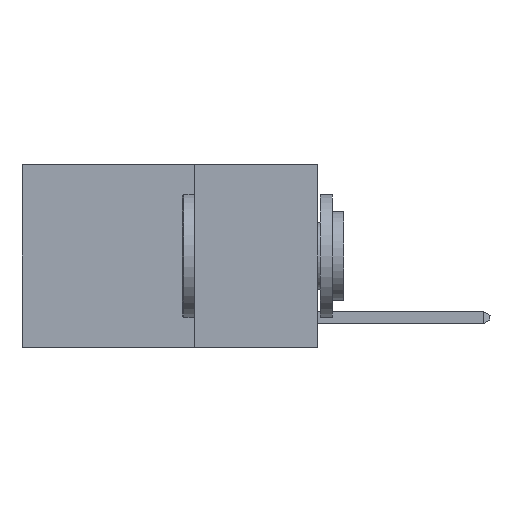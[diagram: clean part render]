
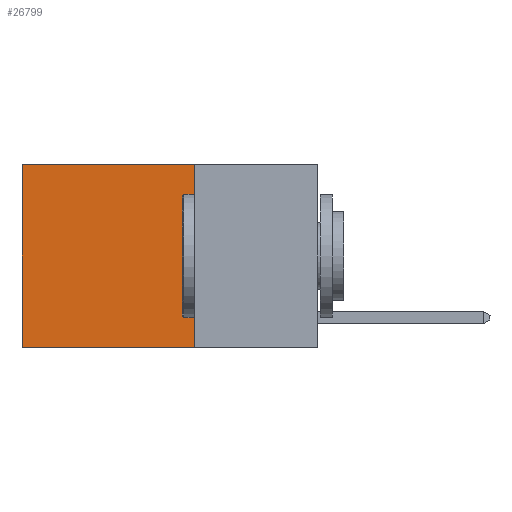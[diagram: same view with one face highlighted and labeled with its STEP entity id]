
A CAD part, left-side view. The second image highlights one B-rep face of the part: STEP entity #26799.
In plain terms, the highlighted planar face has unit normal (-1, 0, 0).
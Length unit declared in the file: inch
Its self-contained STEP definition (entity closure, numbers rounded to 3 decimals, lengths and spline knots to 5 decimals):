
#865 = VERTEX_POINT ( 'NONE', #9514 ) ;
#1272 = CARTESIAN_POINT ( 'NONE',  ( 0.2625, 0.25, -0.37 ) ) ;
#1354 = VECTOR ( 'NONE', #16297, 39.37008 ) ;
#2246 = LINE ( 'NONE', #26280, #8430 ) ;
#4531 = DIRECTION ( 'NONE',  ( 0., 1., 0. ) ) ;
#5643 = VERTEX_POINT ( 'NONE', #23526 ) ;
#7073 = ORIENTED_EDGE ( 'NONE', *, *, #19416, .T. ) ;
#7747 = LINE ( 'NONE', #10006, #25312 ) ;
#8430 = VECTOR ( 'NONE', #4531, 39.37008 ) ;
#8910 = EDGE_CURVE ( 'NONE', #5643, #9985, #27358, .T. ) ;
#9514 = CARTESIAN_POINT ( 'NONE',  ( 0.2625, 0.6, 0. ) ) ;
#9985 = VERTEX_POINT ( 'NONE', #1272 ) ;
#10006 = CARTESIAN_POINT ( 'NONE',  ( 0.2625, 0.25, 0. ) ) ;
#11448 = DIRECTION ( 'NONE',  ( 0., 0., -1. ) ) ;
#13441 = PLANE ( 'NONE',  #13718 ) ;
#13718 = AXIS2_PLACEMENT_3D ( 'NONE', #21730, #15724, #11448 ) ;
#15724 = DIRECTION ( 'NONE',  ( 1., 0., 0. ) ) ;
#16297 = DIRECTION ( 'NONE',  ( 0., 0., -1. ) ) ;
#16443 = DIRECTION ( 'NONE',  ( 0., 1., 0. ) ) ;
#16585 = ORIENTED_EDGE ( 'NONE', *, *, #24616, .T. ) ;
#19061 = CARTESIAN_POINT ( 'NONE',  ( 0.2625, 0.6, -0.37 ) ) ;
#19230 = CARTESIAN_POINT ( 'NONE',  ( 0.2625, 0.6, 0. ) ) ;
#19380 = DIRECTION ( 'NONE',  ( 0., 0., -1. ) ) ;
#19416 = EDGE_CURVE ( 'NONE', #865, #23533, #21373, .T. ) ;
#19991 = ORIENTED_EDGE ( 'NONE', *, *, #23078, .F. ) ;
#21373 = LINE ( 'NONE', #19230, #24421 ) ;
#21730 = CARTESIAN_POINT ( 'NONE',  ( 0.2625, 0.25, 0. ) ) ;
#22682 = ORIENTED_EDGE ( 'NONE', *, *, #8910, .F. ) ;
#23078 = EDGE_CURVE ( 'NONE', #9985, #23533, #2246, .T. ) ;
#23526 = CARTESIAN_POINT ( 'NONE',  ( 0.2625, 0.25, 0. ) ) ;
#23533 = VERTEX_POINT ( 'NONE', #19061 ) ;
#23915 = EDGE_LOOP ( 'NONE', ( #7073, #19991, #22682, #16585 ) ) ;
#24421 = VECTOR ( 'NONE', #19380, 39.37008 ) ;
#24616 = EDGE_CURVE ( 'NONE', #5643, #865, #7747, .T. ) ;
#25312 = VECTOR ( 'NONE', #16443, 39.37008 ) ;
#26280 = CARTESIAN_POINT ( 'NONE',  ( 0.2625, 0.25, -0.37 ) ) ;
#26514 = FACE_OUTER_BOUND ( 'NONE', #23915, .T. ) ;
#26799 = ADVANCED_FACE ( 'NONE', ( #26514 ), #13441, .F. ) ;
#27358 = LINE ( 'NONE', #27498, #1354 ) ;
#27498 = CARTESIAN_POINT ( 'NONE',  ( 0.2625, 0.25, 0. ) ) ;
